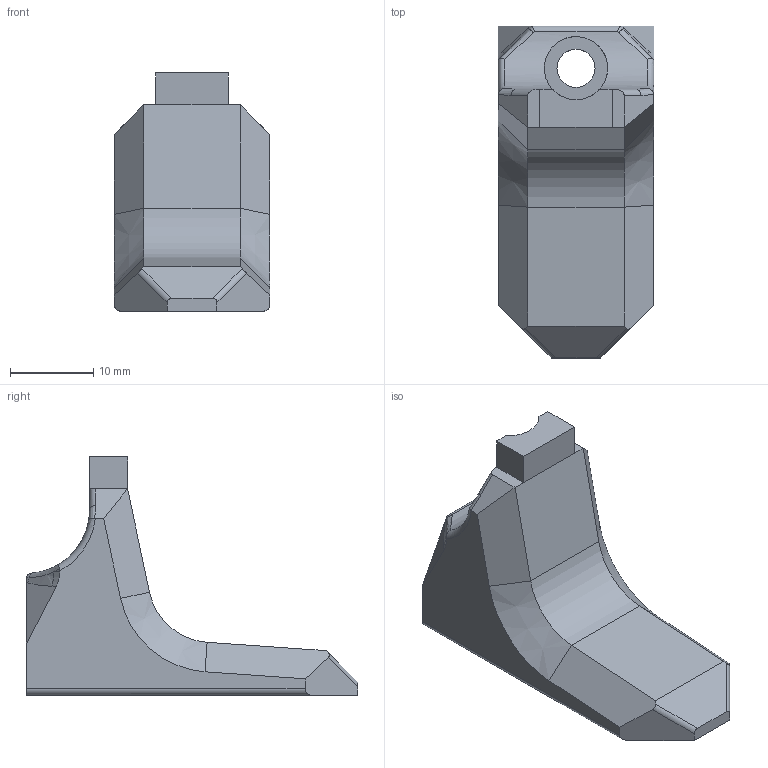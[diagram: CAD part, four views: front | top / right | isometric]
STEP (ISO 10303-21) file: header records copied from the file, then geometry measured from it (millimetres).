
FILE_DESCRIPTION (( 'STEP AP214' ), '1' );
FILE_NAME ('Charging Handle.STEP', '2022-02-04T02:41:23', ( '' ), ( '' ), 'SwSTEP 2.0', 'SolidWorks 2020', '' );
FILE_SCHEMA (( 'AUTOMOTIVE_DESIGN' ));
Length unit declared in the file: inch
Products named in the file (1): Charging Handle
Bounding box: 18.69 x 39.88 x 28.63 mm (x, y, z)
Volume: 6759.6 mm3; surface area: 3110.6 mm2
Topology: 1 solids, 1 shells, 62 faces, 166 edges, 106 vertices
Faces by surface type: plane 33, cylinder 15, bspline 10, cone 2, torus 2
Entity records: 2146 total; most frequent: CARTESIAN_POINT 682, ORIENTED_EDGE 332, DIRECTION 252, EDGE_CURVE 166, VERTEX_POINT 106, LINE 96, VECTOR 96, AXIS2_PLACEMENT_3D 78
